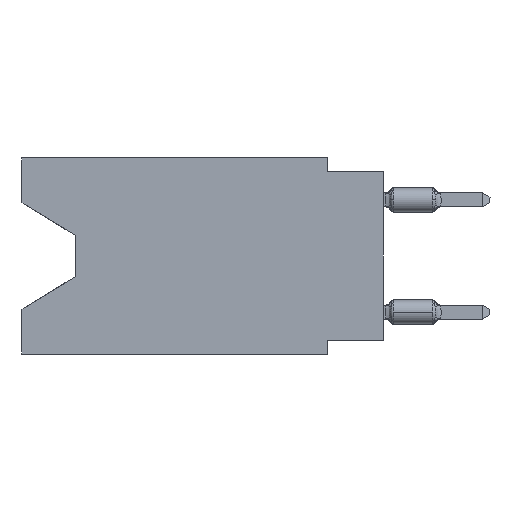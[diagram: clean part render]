
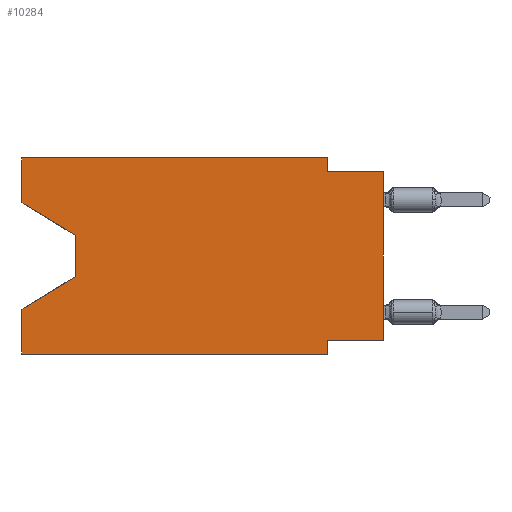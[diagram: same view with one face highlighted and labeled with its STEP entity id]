
A CAD part, left-side view. The second image highlights one B-rep face of the part: STEP entity #10284.
In plain terms, the highlighted planar face has unit normal (-1, 0, 0).
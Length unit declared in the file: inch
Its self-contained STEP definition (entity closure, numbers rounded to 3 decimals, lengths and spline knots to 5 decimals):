
#361 = VECTOR ( 'NONE', #4097, 39.37008 ) ;
#621 = LINE ( 'NONE', #22336, #19680 ) ;
#695 = ORIENTED_EDGE ( 'NONE', *, *, #11916, .F. ) ;
#1018 = EDGE_CURVE ( 'NONE', #8582, #19307, #2808, .T. ) ;
#1021 = CARTESIAN_POINT ( 'NONE',  ( 0., 0., -0.025 ) ) ;
#1043 = VECTOR ( 'NONE', #6171, 39.37008 ) ;
#1484 = EDGE_CURVE ( 'NONE', #11651, #3085, #6223, .T. ) ;
#2104 = CARTESIAN_POINT ( 'NONE',  ( 0., 0., -0.325 ) ) ;
#2486 = LINE ( 'NONE', #13520, #10983 ) ;
#2497 = CARTESIAN_POINT ( 'NONE',  ( 0., 0.645, 0. ) ) ;
#2808 = LINE ( 'NONE', #1021, #6716 ) ;
#3085 = VERTEX_POINT ( 'NONE', #10063 ) ;
#3338 = EDGE_CURVE ( 'NONE', #20320, #16923, #15280, .T. ) ;
#3346 = DIRECTION ( 'NONE',  ( 0., 0., -1. ) ) ;
#3389 = CARTESIAN_POINT ( 'NONE',  ( 0., 0.1, 0. ) ) ;
#4097 = DIRECTION ( 'NONE',  ( 0., 0., -1. ) ) ;
#4361 = LINE ( 'NONE', #11603, #7009 ) ;
#4502 = CARTESIAN_POINT ( 'NONE',  ( 0., 0.645, 0. ) ) ;
#4639 = VERTEX_POINT ( 'NONE', #22565 ) ;
#4674 = CARTESIAN_POINT ( 'NONE',  ( 0., 0.55, -0.212 ) ) ;
#4700 = ORIENTED_EDGE ( 'NONE', *, *, #13512, .F. ) ;
#4818 = VECTOR ( 'NONE', #6351, 39.37008 ) ;
#4819 = EDGE_CURVE ( 'NONE', #12164, #19307, #4361, .T. ) ;
#4947 = ORIENTED_EDGE ( 'NONE', *, *, #22032, .T. ) ;
#5411 = AXIS2_PLACEMENT_3D ( 'NONE', #8245, #17614, #3346 ) ;
#5723 = EDGE_CURVE ( 'NONE', #16923, #11228, #621, .T. ) ;
#6171 = DIRECTION ( 'NONE',  ( 0., -1., 0. ) ) ;
#6223 = LINE ( 'NONE', #11466, #18130 ) ;
#6351 = DIRECTION ( 'NONE',  ( 0., 1., 0. ) ) ;
#6574 = ORIENTED_EDGE ( 'NONE', *, *, #7707, .T. ) ;
#6716 = VECTOR ( 'NONE', #8290, 39.37008 ) ;
#6923 = FACE_OUTER_BOUND ( 'NONE', #13906, .T. ) ;
#6990 = CARTESIAN_POINT ( 'NONE',  ( 0., 0., -0.025 ) ) ;
#7009 = VECTOR ( 'NONE', #7820, 39.37008 ) ;
#7073 = CARTESIAN_POINT ( 'NONE',  ( 0., 0.1, -0.325 ) ) ;
#7280 = VECTOR ( 'NONE', #7974, 39.37008 ) ;
#7707 = EDGE_CURVE ( 'NONE', #11651, #22262, #2486, .T. ) ;
#7742 = VECTOR ( 'NONE', #13501, 39.37008 ) ;
#7820 = DIRECTION ( 'NONE',  ( 0., 0., 1. ) ) ;
#7974 = DIRECTION ( 'NONE',  ( 0., 0., 1. ) ) ;
#8245 = CARTESIAN_POINT ( 'NONE',  ( 0., 0.645, 0. ) ) ;
#8273 = CARTESIAN_POINT ( 'NONE',  ( 0., 0.645, -0.08025 ) ) ;
#8290 = DIRECTION ( 'NONE',  ( 0., -1., 0. ) ) ;
#8382 = DIRECTION ( 'NONE',  ( 0., 0., 1. ) ) ;
#8582 = VERTEX_POINT ( 'NONE', #13543 ) ;
#8959 = ORIENTED_EDGE ( 'NONE', *, *, #22351, .F. ) ;
#9165 = ORIENTED_EDGE ( 'NONE', *, *, #3338, .T. ) ;
#9674 = ORIENTED_EDGE ( 'NONE', *, *, #5723, .T. ) ;
#9684 = VERTEX_POINT ( 'NONE', #7073 ) ;
#9730 = DIRECTION ( 'NONE',  ( 0., -1., 0. ) ) ;
#10063 = CARTESIAN_POINT ( 'NONE',  ( 0., 0.645, -0.26975 ) ) ;
#10098 = ORIENTED_EDGE ( 'NONE', *, *, #1484, .F. ) ;
#10147 = CARTESIAN_POINT ( 'NONE',  ( 0., 0., -0.325 ) ) ;
#10284 = ADVANCED_FACE ( 'NONE', ( #6923 ), #12143, .F. ) ;
#10290 = VECTOR ( 'NONE', #19047, 39.37008 ) ;
#10781 = ORIENTED_EDGE ( 'NONE', *, *, #4819, .T. ) ;
#10983 = VECTOR ( 'NONE', #9730, 39.37008 ) ;
#11102 = CARTESIAN_POINT ( 'NONE',  ( 0., 0.1, 0. ) ) ;
#11228 = VERTEX_POINT ( 'NONE', #12880 ) ;
#11409 = CARTESIAN_POINT ( 'NONE',  ( 0., 0.1, -0.35 ) ) ;
#11466 = CARTESIAN_POINT ( 'NONE',  ( 0., 0.645, 0. ) ) ;
#11603 = CARTESIAN_POINT ( 'NONE',  ( 0., 0., 0. ) ) ;
#11651 = VERTEX_POINT ( 'NONE', #19874 ) ;
#11916 = EDGE_CURVE ( 'NONE', #9684, #22262, #15659, .T. ) ;
#12143 = PLANE ( 'NONE',  #5411 ) ;
#12164 = VERTEX_POINT ( 'NONE', #2104 ) ;
#12880 = CARTESIAN_POINT ( 'NONE',  ( 0., 0.55, -0.212 ) ) ;
#13198 = CARTESIAN_POINT ( 'NONE',  ( 0., 0.645, -0.08025 ) ) ;
#13501 = DIRECTION ( 'NONE',  ( 0., 0., -1. ) ) ;
#13512 = EDGE_CURVE ( 'NONE', #12164, #9684, #18953, .T. ) ;
#13520 = CARTESIAN_POINT ( 'NONE',  ( 0., 0.645, -0.35 ) ) ;
#13543 = CARTESIAN_POINT ( 'NONE',  ( 0., 0.1, -0.025 ) ) ;
#13906 = EDGE_LOOP ( 'NONE', ( #9165, #9674, #4947, #10098, #6574, #695, #4700, #10781, #17269, #15586, #14321, #8959 ) ) ;
#13952 = EDGE_CURVE ( 'NONE', #4639, #19627, #17450, .T. ) ;
#14224 = CARTESIAN_POINT ( 'NONE',  ( 0., 0.55, -0.138 ) ) ;
#14321 = ORIENTED_EDGE ( 'NONE', *, *, #13952, .F. ) ;
#15004 = DIRECTION ( 'NONE',  ( 0., 0., -1. ) ) ;
#15280 = LINE ( 'NONE', #8273, #20396 ) ;
#15586 = ORIENTED_EDGE ( 'NONE', *, *, #19823, .F. ) ;
#15659 = LINE ( 'NONE', #21105, #7742 ) ;
#16923 = VERTEX_POINT ( 'NONE', #14224 ) ;
#17269 = ORIENTED_EDGE ( 'NONE', *, *, #1018, .F. ) ;
#17450 = LINE ( 'NONE', #4502, #1043 ) ;
#17457 = LINE ( 'NONE', #2497, #7280 ) ;
#17614 = DIRECTION ( 'NONE',  ( 1., 0., 0. ) ) ;
#18130 = VECTOR ( 'NONE', #8382, 39.37008 ) ;
#18953 = LINE ( 'NONE', #10147, #4818 ) ;
#19047 = DIRECTION ( 'NONE',  ( 0., 0.855, -0.519 ) ) ;
#19307 = VERTEX_POINT ( 'NONE', #6990 ) ;
#19627 = VERTEX_POINT ( 'NONE', #3389 ) ;
#19680 = VECTOR ( 'NONE', #15004, 39.37008 ) ;
#19823 = EDGE_CURVE ( 'NONE', #19627, #8582, #19911, .T. ) ;
#19874 = CARTESIAN_POINT ( 'NONE',  ( 0., 0.645, -0.35 ) ) ;
#19911 = LINE ( 'NONE', #11102, #361 ) ;
#20320 = VERTEX_POINT ( 'NONE', #13198 ) ;
#20396 = VECTOR ( 'NONE', #22854, 39.37008 ) ;
#21105 = CARTESIAN_POINT ( 'NONE',  ( 0., 0.1, -0.35 ) ) ;
#22032 = EDGE_CURVE ( 'NONE', #11228, #3085, #22575, .T. ) ;
#22262 = VERTEX_POINT ( 'NONE', #11409 ) ;
#22336 = CARTESIAN_POINT ( 'NONE',  ( 0., 0.55, -0.138 ) ) ;
#22351 = EDGE_CURVE ( 'NONE', #20320, #4639, #17457, .T. ) ;
#22565 = CARTESIAN_POINT ( 'NONE',  ( 0., 0.645, 0. ) ) ;
#22575 = LINE ( 'NONE', #4674, #10290 ) ;
#22854 = DIRECTION ( 'NONE',  ( 0., -0.855, -0.519 ) ) ;
